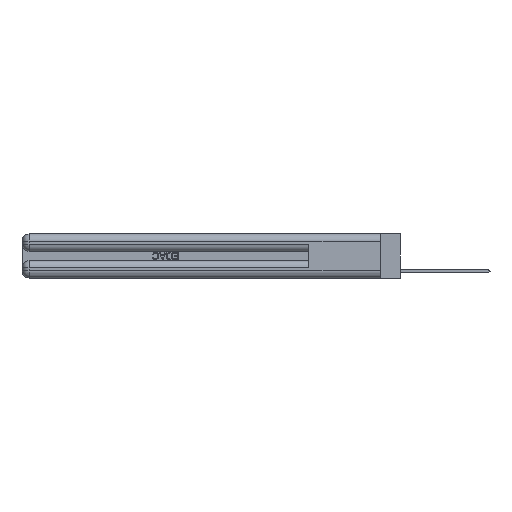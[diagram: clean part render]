
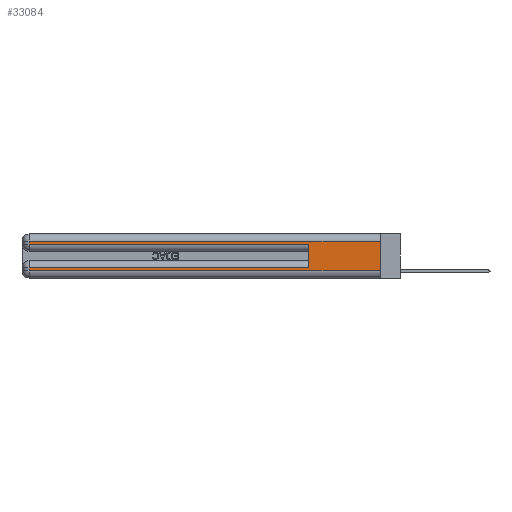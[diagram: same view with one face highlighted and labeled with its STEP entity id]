
A CAD part, left-side view. The second image highlights one B-rep face of the part: STEP entity #33084.
In plain terms, the highlighted planar face has unit normal (-1, 0, 0).
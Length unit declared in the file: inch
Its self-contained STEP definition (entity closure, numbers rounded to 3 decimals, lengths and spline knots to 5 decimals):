
#1556 = ORIENTED_EDGE ( 'NONE', *, *, #26038, .F. ) ;
#2373 = LINE ( 'NONE', #8673, #31458 ) ;
#2632 = EDGE_CURVE ( 'NONE', #11652, #27556, #3364, .T. ) ;
#3050 = CARTESIAN_POINT ( 'NONE',  ( 0., 0., 0.085 ) ) ;
#3364 = LINE ( 'NONE', #5046, #20450 ) ;
#3799 = ORIENTED_EDGE ( 'NONE', *, *, #15596, .T. ) ;
#4103 = VERTEX_POINT ( 'NONE', #10012 ) ;
#4155 = LINE ( 'NONE', #10983, #8443 ) ;
#4786 = FACE_OUTER_BOUND ( 'NONE', #8660, .T. ) ;
#4894 = CARTESIAN_POINT ( 'NONE',  ( 0., 0.6, 0.285 ) ) ;
#5046 = CARTESIAN_POINT ( 'NONE',  ( 0., 0., 0.31 ) ) ;
#5159 = VECTOR ( 'NONE', #5814, 39.37008 ) ;
#5814 = DIRECTION ( 'NONE',  ( 0., -1., 0. ) ) ;
#6896 = CARTESIAN_POINT ( 'NONE',  ( 0., 2.94, 0.31 ) ) ;
#8067 = CARTESIAN_POINT ( 'NONE',  ( 0., 0.6, 0.085 ) ) ;
#8443 = VECTOR ( 'NONE', #14041, 39.37008 ) ;
#8488 = ORIENTED_EDGE ( 'NONE', *, *, #8970, .T. ) ;
#8569 = DIRECTION ( 'NONE',  ( 0., 1., 0. ) ) ;
#8660 = EDGE_LOOP ( 'NONE', ( #1556, #23868, #26313, #11193, #27435, #8488, #10821, #3799 ) ) ;
#8673 = CARTESIAN_POINT ( 'NONE',  ( 0., 0.6, 0.145 ) ) ;
#8970 = EDGE_CURVE ( 'NONE', #34902, #12437, #11162, .T. ) ;
#10012 = CARTESIAN_POINT ( 'NONE',  ( 0., 2.94, 0.06 ) ) ;
#10029 = AXIS2_PLACEMENT_3D ( 'NONE', #24227, #32098, #18478 ) ;
#10821 = ORIENTED_EDGE ( 'NONE', *, *, #18752, .T. ) ;
#10983 = CARTESIAN_POINT ( 'NONE',  ( 0., 0., 0.285 ) ) ;
#10996 = VECTOR ( 'NONE', #35033, 39.37008 ) ;
#11162 = LINE ( 'NONE', #3050, #12852 ) ;
#11193 = ORIENTED_EDGE ( 'NONE', *, *, #29180, .T. ) ;
#11652 = VERTEX_POINT ( 'NONE', #15955 ) ;
#12068 = CARTESIAN_POINT ( 'NONE',  ( 0., 2.94, 0.37 ) ) ;
#12437 = VERTEX_POINT ( 'NONE', #27752 ) ;
#12852 = VECTOR ( 'NONE', #8569, 39.37008 ) ;
#13023 = EDGE_CURVE ( 'NONE', #34902, #23132, #2373, .T. ) ;
#13068 = LINE ( 'NONE', #12068, #14783 ) ;
#14041 = DIRECTION ( 'NONE',  ( 0., -1., 0. ) ) ;
#14783 = VECTOR ( 'NONE', #28939, 39.37008 ) ;
#15596 = EDGE_CURVE ( 'NONE', #4103, #32010, #29110, .T. ) ;
#15698 = PLANE ( 'NONE',  #10029 ) ;
#15826 = DIRECTION ( 'NONE',  ( 0., 0., -1. ) ) ;
#15937 = CARTESIAN_POINT ( 'NONE',  ( 0., 0., 0.37 ) ) ;
#15955 = CARTESIAN_POINT ( 'NONE',  ( 0., 0., 0.31 ) ) ;
#16175 = EDGE_CURVE ( 'NONE', #27556, #30616, #21341, .T. ) ;
#16531 = LINE ( 'NONE', #15937, #10996 ) ;
#18478 = DIRECTION ( 'NONE',  ( 0., 0., -1. ) ) ;
#18752 = EDGE_CURVE ( 'NONE', #12437, #4103, #13068, .T. ) ;
#19228 = DIRECTION ( 'NONE',  ( 0., 1., 0. ) ) ;
#20450 = VECTOR ( 'NONE', #19228, 39.37008 ) ;
#21289 = CARTESIAN_POINT ( 'NONE',  ( 0., 0., 0.06 ) ) ;
#21341 = LINE ( 'NONE', #29367, #33686 ) ;
#22024 = DIRECTION ( 'NONE',  ( 0., 0., 1. ) ) ;
#23132 = VERTEX_POINT ( 'NONE', #4894 ) ;
#23868 = ORIENTED_EDGE ( 'NONE', *, *, #2632, .T. ) ;
#24044 = CARTESIAN_POINT ( 'NONE',  ( 0., 2.94, 0.285 ) ) ;
#24227 = CARTESIAN_POINT ( 'NONE',  ( 0., 0., 0.37 ) ) ;
#26038 = EDGE_CURVE ( 'NONE', #11652, #32010, #16531, .T. ) ;
#26313 = ORIENTED_EDGE ( 'NONE', *, *, #16175, .T. ) ;
#27435 = ORIENTED_EDGE ( 'NONE', *, *, #13023, .F. ) ;
#27556 = VERTEX_POINT ( 'NONE', #6896 ) ;
#27752 = CARTESIAN_POINT ( 'NONE',  ( 0., 2.94, 0.085 ) ) ;
#28939 = DIRECTION ( 'NONE',  ( 0., 0., -1. ) ) ;
#29110 = LINE ( 'NONE', #30163, #5159 ) ;
#29180 = EDGE_CURVE ( 'NONE', #30616, #23132, #4155, .T. ) ;
#29367 = CARTESIAN_POINT ( 'NONE',  ( 0., 2.94, 0.37 ) ) ;
#30163 = CARTESIAN_POINT ( 'NONE',  ( 0., 0., 0.06 ) ) ;
#30616 = VERTEX_POINT ( 'NONE', #24044 ) ;
#31458 = VECTOR ( 'NONE', #22024, 39.37008 ) ;
#32010 = VERTEX_POINT ( 'NONE', #21289 ) ;
#32098 = DIRECTION ( 'NONE',  ( 1., 0., 0. ) ) ;
#33084 = ADVANCED_FACE ( 'NONE', ( #4786 ), #15698, .F. ) ;
#33686 = VECTOR ( 'NONE', #15826, 39.37008 ) ;
#34902 = VERTEX_POINT ( 'NONE', #8067 ) ;
#35033 = DIRECTION ( 'NONE',  ( 0., 0., -1. ) ) ;
